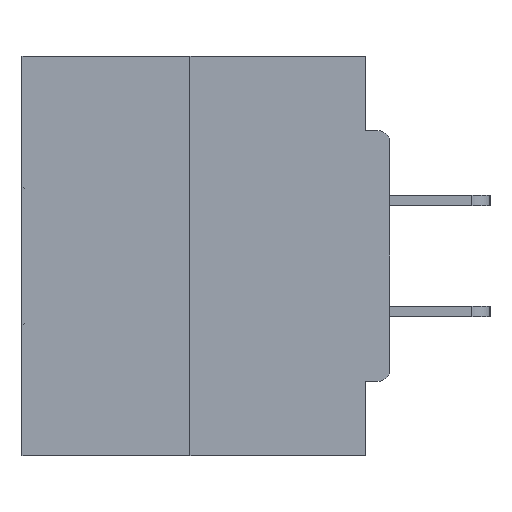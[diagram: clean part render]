
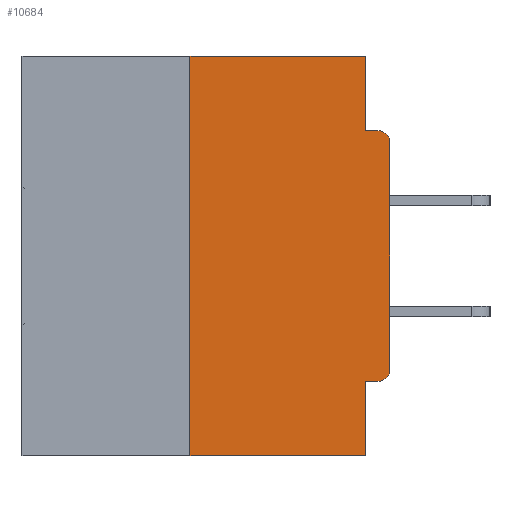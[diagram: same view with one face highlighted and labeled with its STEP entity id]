
A CAD part, left-side view. The second image highlights one B-rep face of the part: STEP entity #10684.
In plain terms, the highlighted planar face has unit normal (-1, 0, 0).
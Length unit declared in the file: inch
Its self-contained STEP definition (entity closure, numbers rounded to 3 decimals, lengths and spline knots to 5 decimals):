
#119 = EDGE_CURVE ( 'NONE', #2206, #11494, #8906, .T. ) ;
#385 = DIRECTION ( 'NONE',  ( -1., 0., 0. ) ) ;
#471 = ORIENTED_EDGE ( 'NONE', *, *, #32772, .T. ) ;
#1501 = AXIS2_PLACEMENT_3D ( 'NONE', #28120, #385, #11936 ) ;
#1788 = EDGE_LOOP ( 'NONE', ( #9310, #15018, #29565, #6431, #6542, #4503, #9418, #471, #17078, #12285 ) ) ;
#2206 = VERTEX_POINT ( 'NONE', #23547 ) ;
#2625 = DIRECTION ( 'NONE',  ( 0., 0., -1. ) ) ;
#2833 = CARTESIAN_POINT ( 'NONE',  ( 0., 0.031, -0.0935 ) ) ;
#3744 = CARTESIAN_POINT ( 'NONE',  ( 0., 0.25, 0. ) ) ;
#4503 = ORIENTED_EDGE ( 'NONE', *, *, #9967, .T. ) ;
#4714 = CIRCLE ( 'NONE', #1501, 0.015 ) ;
#5731 = CARTESIAN_POINT ( 'NONE',  ( 0., 0.46, 0. ) ) ;
#5874 = CARTESIAN_POINT ( 'NONE',  ( 0., 0.031, 0. ) ) ;
#6087 = DIRECTION ( 'NONE',  ( 1., 0., 0. ) ) ;
#6213 = DIRECTION ( 'NONE',  ( 0., 0., 1. ) ) ;
#6431 = ORIENTED_EDGE ( 'NONE', *, *, #8408, .F. ) ;
#6542 = ORIENTED_EDGE ( 'NONE', *, *, #33283, .F. ) ;
#7454 = VECTOR ( 'NONE', #18266, 39.37008 ) ;
#7617 = CARTESIAN_POINT ( 'NONE',  ( 0., 0.031, -0.5 ) ) ;
#7799 = VECTOR ( 'NONE', #6213, 39.37008 ) ;
#8408 = EDGE_CURVE ( 'NONE', #11514, #23045, #16342, .T. ) ;
#8414 = VECTOR ( 'NONE', #16325, 39.37008 ) ;
#8482 = CARTESIAN_POINT ( 'NONE',  ( 0., 0.031, -0.4065 ) ) ;
#8702 = PLANE ( 'NONE',  #35394 ) ;
#8846 = VERTEX_POINT ( 'NONE', #3744 ) ;
#8906 = LINE ( 'NONE', #5874, #32728 ) ;
#9239 = LINE ( 'NONE', #15332, #7799 ) ;
#9310 = ORIENTED_EDGE ( 'NONE', *, *, #30686, .F. ) ;
#9418 = ORIENTED_EDGE ( 'NONE', *, *, #21938, .T. ) ;
#9764 = VECTOR ( 'NONE', #11288, 39.37008 ) ;
#9967 = EDGE_CURVE ( 'NONE', #35562, #33918, #28230, .T. ) ;
#10014 = DIRECTION ( 'NONE',  ( -1., 0., 0. ) ) ;
#10211 = DIRECTION ( 'NONE',  ( 0., 0., -1. ) ) ;
#10451 = LINE ( 'NONE', #16531, #8414 ) ;
#10684 = ADVANCED_FACE ( 'NONE', ( #15201 ), #8702, .F. ) ;
#10883 = VERTEX_POINT ( 'NONE', #37661 ) ;
#11288 = DIRECTION ( 'NONE',  ( 0., -1., 0. ) ) ;
#11415 = EDGE_CURVE ( 'NONE', #11494, #10883, #10451, .T. ) ;
#11494 = VERTEX_POINT ( 'NONE', #2833 ) ;
#11514 = VERTEX_POINT ( 'NONE', #8482 ) ;
#11557 = DIRECTION ( 'NONE',  ( 0., 0., -1. ) ) ;
#11636 = CARTESIAN_POINT ( 'NONE',  ( 0., 0.25, -0.5 ) ) ;
#11936 = DIRECTION ( 'NONE',  ( 0., 0., -1. ) ) ;
#12285 = ORIENTED_EDGE ( 'NONE', *, *, #119, .F. ) ;
#12725 = AXIS2_PLACEMENT_3D ( 'NONE', #26700, #10014, #10211 ) ;
#13272 = CARTESIAN_POINT ( 'NONE',  ( 0., 0., -0.4065 ) ) ;
#14716 = LINE ( 'NONE', #27059, #9764 ) ;
#15018 = ORIENTED_EDGE ( 'NONE', *, *, #27827, .F. ) ;
#15201 = FACE_OUTER_BOUND ( 'NONE', #1788, .T. ) ;
#15332 = CARTESIAN_POINT ( 'NONE',  ( 0., 0.25, 0. ) ) ;
#16325 = DIRECTION ( 'NONE',  ( 0., -1., 0. ) ) ;
#16342 = LINE ( 'NONE', #37832, #21671 ) ;
#16531 = CARTESIAN_POINT ( 'NONE',  ( 0., 0., -0.0935 ) ) ;
#17078 = ORIENTED_EDGE ( 'NONE', *, *, #11415, .F. ) ;
#17883 = LINE ( 'NONE', #33662, #7454 ) ;
#18243 = VECTOR ( 'NONE', #30022, 39.37008 ) ;
#18266 = DIRECTION ( 'NONE',  ( 0., 0., 1. ) ) ;
#20059 = CARTESIAN_POINT ( 'NONE',  ( 0., 0., -0.3915 ) ) ;
#21399 = CARTESIAN_POINT ( 'NONE',  ( 0., 0., -0.1085 ) ) ;
#21671 = VECTOR ( 'NONE', #38026, 39.37008 ) ;
#21938 = EDGE_CURVE ( 'NONE', #33918, #39609, #17883, .T. ) ;
#23045 = VERTEX_POINT ( 'NONE', #7617 ) ;
#23547 = CARTESIAN_POINT ( 'NONE',  ( 0., 0.031, 0. ) ) ;
#26700 = CARTESIAN_POINT ( 'NONE',  ( 0., 0.015, -0.3915 ) ) ;
#27059 = CARTESIAN_POINT ( 'NONE',  ( 0., 0.46, -0.5 ) ) ;
#27744 = EDGE_CURVE ( 'NONE', #30307, #23045, #14716, .T. ) ;
#27827 = EDGE_CURVE ( 'NONE', #30307, #8846, #9239, .T. ) ;
#28120 = CARTESIAN_POINT ( 'NONE',  ( 0., 0.015, -0.1085 ) ) ;
#28230 = CIRCLE ( 'NONE', #12725, 0.015 ) ;
#29565 = ORIENTED_EDGE ( 'NONE', *, *, #27744, .T. ) ;
#30022 = DIRECTION ( 'NONE',  ( 0., -1., 0. ) ) ;
#30163 = CARTESIAN_POINT ( 'NONE',  ( 0., 0.015, -0.4065 ) ) ;
#30307 = VERTEX_POINT ( 'NONE', #11636 ) ;
#30627 = VECTOR ( 'NONE', #37569, 39.37008 ) ;
#30686 = EDGE_CURVE ( 'NONE', #8846, #2206, #35899, .T. ) ;
#32728 = VECTOR ( 'NONE', #11557, 39.37008 ) ;
#32772 = EDGE_CURVE ( 'NONE', #39609, #10883, #4714, .T. ) ;
#33283 = EDGE_CURVE ( 'NONE', #35562, #11514, #34538, .T. ) ;
#33662 = CARTESIAN_POINT ( 'NONE',  ( 0., 0., 0. ) ) ;
#33918 = VERTEX_POINT ( 'NONE', #20059 ) ;
#34538 = LINE ( 'NONE', #13272, #30627 ) ;
#35394 = AXIS2_PLACEMENT_3D ( 'NONE', #39917, #6087, #2625 ) ;
#35562 = VERTEX_POINT ( 'NONE', #30163 ) ;
#35899 = LINE ( 'NONE', #5731, #18243 ) ;
#37569 = DIRECTION ( 'NONE',  ( 0., 1., 0. ) ) ;
#37661 = CARTESIAN_POINT ( 'NONE',  ( 0., 0.015, -0.0935 ) ) ;
#37832 = CARTESIAN_POINT ( 'NONE',  ( 0., 0.031, -0.5 ) ) ;
#38026 = DIRECTION ( 'NONE',  ( 0., 0., -1. ) ) ;
#39609 = VERTEX_POINT ( 'NONE', #21399 ) ;
#39917 = CARTESIAN_POINT ( 'NONE',  ( 0., 0.46, 0. ) ) ;
